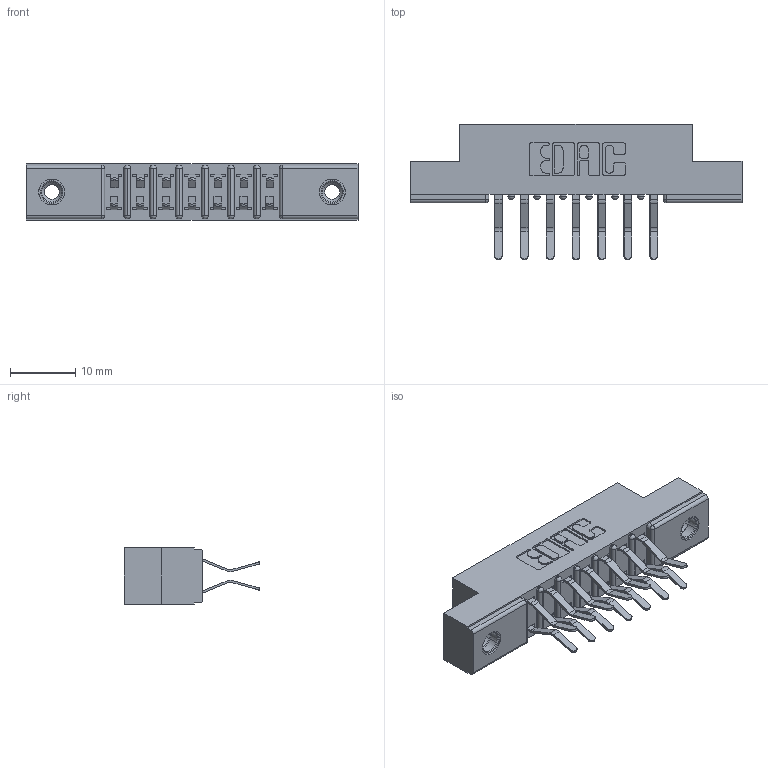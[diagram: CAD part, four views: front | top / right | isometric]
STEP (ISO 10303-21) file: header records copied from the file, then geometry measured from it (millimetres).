
FILE_DESCRIPTION (( 'STEP AP203' ), '1' );
FILE_NAME ('307-014-460-208.STEP', '2020-09-28T16:38:35', ( '' ), ( '' ), 'SwSTEP 2.0', 'SolidWorks 2020', '' );
FILE_SCHEMA (( 'CONFIG_CONTROL_DESIGN' ));
Length unit declared in the file: inch
Products named in the file (4): 307 Part_.156 Dia Mounting Holes; 307-014-460-208; 307-290-001_560; 345-250-001_345-250-003-102
Assembly tree (17 placements, depth 2):
  307-014-460-208
    307 Part_.156 Dia Mounting Holes
    307-290-001_560  x14
    345-250-001_345-250-003-102  x2
Bounding box: 50.75 x 20.73 x 8.71 mm (x, y, z)
Volume: 3332.2 mm3; surface area: 5230.8 mm2
Topology: 17 solids, 17 shells, 886 faces, 2447 edges, 1582 vertices
Faces by surface type: plane 564, cylinder 290, sphere 16, cone 12, torus 4
Entity records: 11829 total; most frequent: CARTESIAN_POINT 1930, DIRECTION 1915, ORIENTED_EDGE 1902, EDGE_CURVE 951, VECTOR 713, LINE 713, VERTEX_POINT 616, AXIS2_PLACEMENT_3D 601
